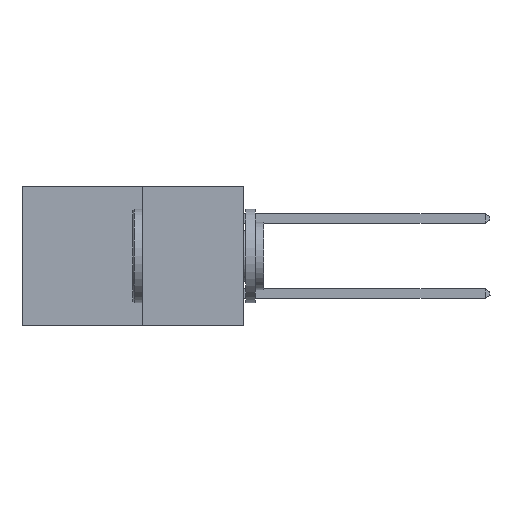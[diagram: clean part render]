
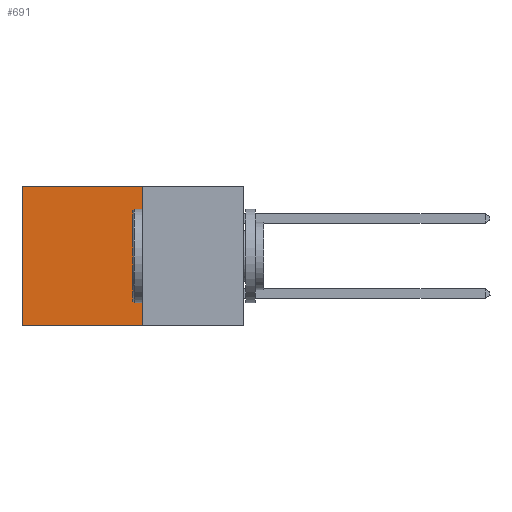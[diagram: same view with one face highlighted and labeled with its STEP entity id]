
A CAD part, left-side view. The second image highlights one B-rep face of the part: STEP entity #691.
In plain terms, the highlighted planar face has unit normal (-1, 0, 0).
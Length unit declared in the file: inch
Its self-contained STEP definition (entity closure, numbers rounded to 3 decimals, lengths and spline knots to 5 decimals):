
#2 = LINE ( 'NONE', #7164, #10258 ) ;
#278 = VERTEX_POINT ( 'NONE', #3708 ) ;
#421 = EDGE_CURVE ( 'NONE', #5349, #5109, #2960, .T. ) ;
#691 = ADVANCED_FACE ( 'NONE', ( #7119 ), #6164, .F. ) ;
#783 = CARTESIAN_POINT ( 'NONE',  ( 0.277, 0.59, -0.37 ) ) ;
#795 = VECTOR ( 'NONE', #6346, 39.37008 ) ;
#1335 = AXIS2_PLACEMENT_3D ( 'NONE', #6796, #2649, #4568 ) ;
#1469 = EDGE_CURVE ( 'NONE', #278, #5109, #2, .T. ) ;
#1552 = VECTOR ( 'NONE', #9096, 39.37008 ) ;
#2649 = DIRECTION ( 'NONE',  ( 1., 0., 0. ) ) ;
#2960 = LINE ( 'NONE', #3508, #795 ) ;
#3011 = DIRECTION ( 'NONE',  ( 0., 1., 0. ) ) ;
#3508 = CARTESIAN_POINT ( 'NONE',  ( 0.277, 0.59, -0.37 ) ) ;
#3697 = CARTESIAN_POINT ( 'NONE',  ( 0.277, 0.27, 0. ) ) ;
#3708 = CARTESIAN_POINT ( 'NONE',  ( 0.277, 0.27, -0.37 ) ) ;
#3712 = LINE ( 'NONE', #4340, #1552 ) ;
#3864 = ORIENTED_EDGE ( 'NONE', *, *, #421, .T. ) ;
#4340 = CARTESIAN_POINT ( 'NONE',  ( 0.277, 0.27, -0.37 ) ) ;
#4553 = ORIENTED_EDGE ( 'NONE', *, *, #9500, .F. ) ;
#4568 = DIRECTION ( 'NONE',  ( 0., 0., -1. ) ) ;
#4816 = ORIENTED_EDGE ( 'NONE', *, *, #6009, .T. ) ;
#5109 = VERTEX_POINT ( 'NONE', #783 ) ;
#5349 = VERTEX_POINT ( 'NONE', #10058 ) ;
#6001 = VECTOR ( 'NONE', #3011, 39.37008 ) ;
#6009 = EDGE_CURVE ( 'NONE', #7947, #5349, #8111, .T. ) ;
#6164 = PLANE ( 'NONE',  #1335 ) ;
#6188 = CARTESIAN_POINT ( 'NONE',  ( 0.277, 0.27, 0. ) ) ;
#6346 = DIRECTION ( 'NONE',  ( 0., 0., -1. ) ) ;
#6796 = CARTESIAN_POINT ( 'NONE',  ( 0.277, 0.27, -0.37 ) ) ;
#7119 = FACE_OUTER_BOUND ( 'NONE', #9695, .T. ) ;
#7164 = CARTESIAN_POINT ( 'NONE',  ( 0.277, 0.27, -0.37 ) ) ;
#7947 = VERTEX_POINT ( 'NONE', #6188 ) ;
#8111 = LINE ( 'NONE', #3697, #6001 ) ;
#9096 = DIRECTION ( 'NONE',  ( 0., 0., -1. ) ) ;
#9334 = DIRECTION ( 'NONE',  ( 0., 1., 0. ) ) ;
#9500 = EDGE_CURVE ( 'NONE', #7947, #278, #3712, .T. ) ;
#9695 = EDGE_LOOP ( 'NONE', ( #3864, #10410, #4553, #4816 ) ) ;
#10058 = CARTESIAN_POINT ( 'NONE',  ( 0.277, 0.59, 0. ) ) ;
#10258 = VECTOR ( 'NONE', #9334, 39.37008 ) ;
#10410 = ORIENTED_EDGE ( 'NONE', *, *, #1469, .F. ) ;
